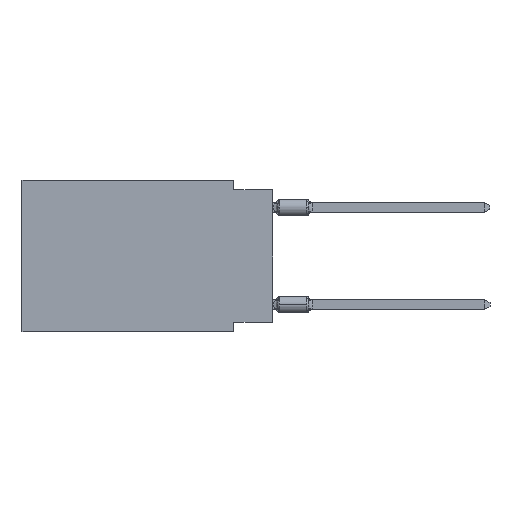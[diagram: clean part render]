
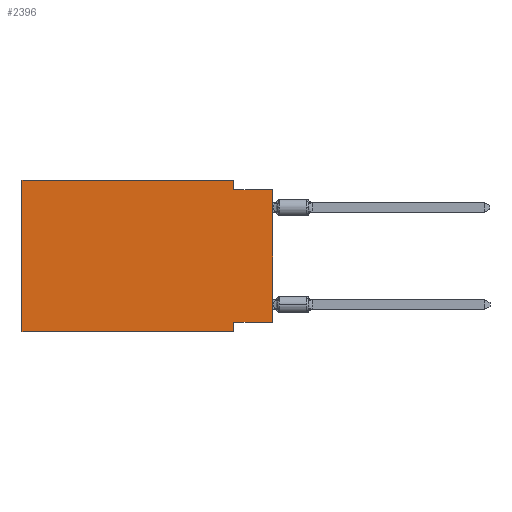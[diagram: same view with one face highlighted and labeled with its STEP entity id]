
A CAD part, left-side view. The second image highlights one B-rep face of the part: STEP entity #2396.
In plain terms, the highlighted planar face has unit normal (-1, 0, 0).
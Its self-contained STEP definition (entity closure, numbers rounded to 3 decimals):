
#82 = CARTESIAN_POINT ( 'NONE',  ( 0., 16.383, -9.906 ) ) ;
#371 = VECTOR ( 'NONE', #10370, 1000. ) ;
#824 = EDGE_CURVE ( 'NONE', #19501, #1407, #9421, .T. ) ;
#884 = FACE_OUTER_BOUND ( 'NONE', #19033, .T. ) ;
#890 = CARTESIAN_POINT ( 'NONE',  ( 0., 2.54, -9.906 ) ) ;
#1080 = ORIENTED_EDGE ( 'NONE', *, *, #824, .F. ) ;
#1111 = DIRECTION ( 'NONE',  ( 0., 0., -1. ) ) ;
#1240 = VECTOR ( 'NONE', #7943, 1000. ) ;
#1407 = VERTEX_POINT ( 'NONE', #3181 ) ;
#1721 = VERTEX_POINT ( 'NONE', #13418 ) ;
#1929 = CARTESIAN_POINT ( 'NONE',  ( 0., 0., -9.271 ) ) ;
#2138 = CARTESIAN_POINT ( 'NONE',  ( 0., 0., -9.271 ) ) ;
#2366 = EDGE_CURVE ( 'NONE', #1407, #1721, #22691, .T. ) ;
#2396 = ADVANCED_FACE ( 'NONE', ( #884 ), #13224, .F. ) ;
#2509 = CARTESIAN_POINT ( 'NONE',  ( 0., 16.383, 0. ) ) ;
#3033 = EDGE_CURVE ( 'NONE', #1721, #11647, #12318, .T. ) ;
#3181 = CARTESIAN_POINT ( 'NONE',  ( 0., 2.54, 0. ) ) ;
#3737 = CARTESIAN_POINT ( 'NONE',  ( 0., 16.383, 0. ) ) ;
#3739 = CARTESIAN_POINT ( 'NONE',  ( 0., 16.383, 0. ) ) ;
#3860 = DIRECTION ( 'NONE',  ( 0., 0., 1. ) ) ;
#3969 = ORIENTED_EDGE ( 'NONE', *, *, #9696, .T. ) ;
#4362 = CARTESIAN_POINT ( 'NONE',  ( 0., 2.54, -9.906 ) ) ;
#4496 = DIRECTION ( 'NONE',  ( 0., -1., 0. ) ) ;
#4774 = VECTOR ( 'NONE', #4496, 1000. ) ;
#5366 = CARTESIAN_POINT ( 'NONE',  ( 0., 2.54, -9.271 ) ) ;
#5407 = DIRECTION ( 'NONE',  ( 0., 1., 0. ) ) ;
#5646 = CARTESIAN_POINT ( 'NONE',  ( 0., 16.383, 0. ) ) ;
#5833 = ORIENTED_EDGE ( 'NONE', *, *, #11418, .T. ) ;
#6500 = DIRECTION ( 'NONE',  ( 0., 0., 1. ) ) ;
#7823 = DIRECTION ( 'NONE',  ( 0., 0., -1. ) ) ;
#7943 = DIRECTION ( 'NONE',  ( 0., 0., -1. ) ) ;
#8556 = CARTESIAN_POINT ( 'NONE',  ( 0., 0., 0. ) ) ;
#8573 = VECTOR ( 'NONE', #21705, 1000. ) ;
#9333 = LINE ( 'NONE', #1929, #11657 ) ;
#9421 = LINE ( 'NONE', #3739, #8573 ) ;
#9696 = EDGE_CURVE ( 'NONE', #15738, #11647, #13720, .T. ) ;
#9697 = CARTESIAN_POINT ( 'NONE',  ( 0., 16.383, -9.906 ) ) ;
#10237 = ORIENTED_EDGE ( 'NONE', *, *, #2366, .F. ) ;
#10370 = DIRECTION ( 'NONE',  ( 0., -1., 0. ) ) ;
#11418 = EDGE_CURVE ( 'NONE', #11720, #15464, #14880, .T. ) ;
#11647 = VERTEX_POINT ( 'NONE', #14388 ) ;
#11657 = VECTOR ( 'NONE', #5407, 1000. ) ;
#11720 = VERTEX_POINT ( 'NONE', #82 ) ;
#12261 = ORIENTED_EDGE ( 'NONE', *, *, #21520, .F. ) ;
#12273 = ORIENTED_EDGE ( 'NONE', *, *, #22690, .F. ) ;
#12318 = LINE ( 'NONE', #19212, #371 ) ;
#13159 = LINE ( 'NONE', #3737, #14151 ) ;
#13224 = PLANE ( 'NONE',  #17076 ) ;
#13418 = CARTESIAN_POINT ( 'NONE',  ( 0., 2.54, -0.635 ) ) ;
#13720 = LINE ( 'NONE', #8556, #18061 ) ;
#13911 = ORIENTED_EDGE ( 'NONE', *, *, #15370, .F. ) ;
#14151 = VECTOR ( 'NONE', #3860, 1000. ) ;
#14388 = CARTESIAN_POINT ( 'NONE',  ( 0., 0., -0.635 ) ) ;
#14880 = LINE ( 'NONE', #9697, #4774 ) ;
#14964 = CARTESIAN_POINT ( 'NONE',  ( 0., 2.54, 0. ) ) ;
#15370 = EDGE_CURVE ( 'NONE', #21377, #15464, #18746, .T. ) ;
#15464 = VERTEX_POINT ( 'NONE', #890 ) ;
#15577 = ORIENTED_EDGE ( 'NONE', *, *, #3033, .F. ) ;
#15738 = VERTEX_POINT ( 'NONE', #2138 ) ;
#17076 = AXIS2_PLACEMENT_3D ( 'NONE', #2509, #20239, #7823 ) ;
#17986 = VECTOR ( 'NONE', #1111, 1000. ) ;
#18061 = VECTOR ( 'NONE', #6500, 1000. ) ;
#18746 = LINE ( 'NONE', #4362, #17986 ) ;
#19033 = EDGE_LOOP ( 'NONE', ( #3969, #15577, #10237, #1080, #12261, #5833, #13911, #12273 ) ) ;
#19212 = CARTESIAN_POINT ( 'NONE',  ( 0., 0., -0.635 ) ) ;
#19501 = VERTEX_POINT ( 'NONE', #5646 ) ;
#20239 = DIRECTION ( 'NONE',  ( 1., 0., 0. ) ) ;
#21377 = VERTEX_POINT ( 'NONE', #5366 ) ;
#21520 = EDGE_CURVE ( 'NONE', #11720, #19501, #13159, .T. ) ;
#21705 = DIRECTION ( 'NONE',  ( 0., -1., 0. ) ) ;
#22690 = EDGE_CURVE ( 'NONE', #15738, #21377, #9333, .T. ) ;
#22691 = LINE ( 'NONE', #14964, #1240 ) ;
